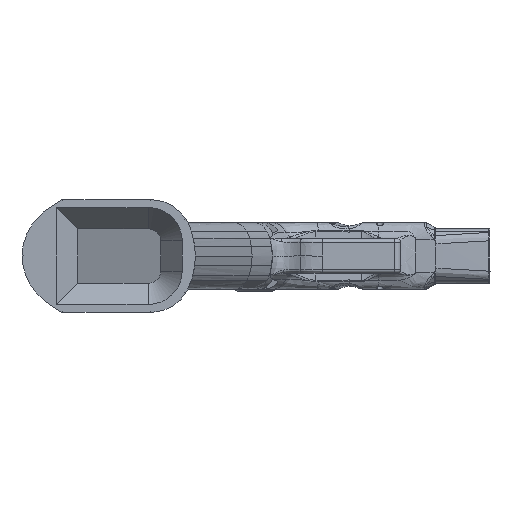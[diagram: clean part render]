
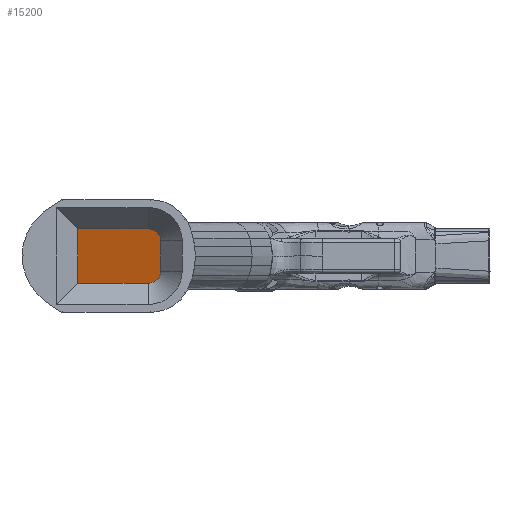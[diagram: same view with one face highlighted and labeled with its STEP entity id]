
A CAD part, front view. The second image highlights one B-rep face of the part: STEP entity #15200.
In plain terms, the highlighted planar face has unit normal (0.951, -0.309, 0).
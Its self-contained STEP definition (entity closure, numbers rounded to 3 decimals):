
#685 = CARTESIAN_POINT ( 'NONE',  ( 32.169, -5.875, -11.75 ) ) ;
#763 = EDGE_CURVE ( 'NONE', #20074, #12937, #11193, .T. ) ;
#1155 = VECTOR ( 'NONE', #11924, 1000. ) ;
#1711 = VECTOR ( 'NONE', #37430, 1000. ) ;
#1753 = LINE ( 'NONE', #5412, #18386 ) ;
#2363 = ORIENTED_EDGE ( 'NONE', *, *, #28812, .F. ) ;
#2663 = CARTESIAN_POINT ( 'NONE',  ( 32.169, -5.875, -11.75 ) ) ;
#3566 = VERTEX_POINT ( 'NONE', #685 ) ;
#4334 = VERTEX_POINT ( 'NONE', #40882 ) ;
#5311 = CARTESIAN_POINT ( 'NONE',  ( -22.8, -175.052, 11.75 ) ) ;
#5412 = CARTESIAN_POINT ( 'NONE',  ( -22.8, -175.052, -11.75 ) ) ;
#7795 = CARTESIAN_POINT ( 'NONE',  ( 32.169, -5.875, -11.75 ) ) ;
#8063 = VECTOR ( 'NONE', #37398, 1000. ) ;
#8209 = DIRECTION ( 'NONE',  ( 0.309, 0.951, 0. ) ) ;
#8543 = ORIENTED_EDGE ( 'NONE', *, *, #13688, .T. ) ;
#8795 = VERTEX_POINT ( 'NONE', #20114 ) ;
#8968 = ORIENTED_EDGE ( 'NONE', *, *, #29911, .F. ) ;
#9107 = DIRECTION ( 'NONE',  ( 0., 0., 1. ) ) ;
#10800 = VECTOR ( 'NONE', #22434, 1000. ) ;
#11193 = LINE ( 'NONE', #24298, #8063 ) ;
#11903 = LINE ( 'NONE', #41331, #29871 ) ;
#11924 = DIRECTION ( 'NONE',  ( -0.309, -0.951, 0. ) ) ;
#12059 = LINE ( 'NONE', #34624, #29429 ) ;
#12372 = VERTEX_POINT ( 'NONE', #12800 ) ;
#12542 = ORIENTED_EDGE ( 'NONE', *, *, #29637, .T. ) ;
#12647 = DIRECTION ( 'NONE',  ( -0.951, 0.309, 0. ) ) ;
#12800 = CARTESIAN_POINT ( 'NONE',  ( 33.591, -1.5, -10.375 ) ) ;
#12937 = VERTEX_POINT ( 'NONE', #38001 ) ;
#13088 = CARTESIAN_POINT ( 'NONE',  ( 2.312, -97.765, -11.75 ) ) ;
#13688 = EDGE_CURVE ( 'NONE', #12372, #33228, #11903, .T. ) ;
#13911 = EDGE_CURVE ( 'NONE', #3566, #4334, #30365, .T. ) ;
#15200 = ADVANCED_FACE ( 'NONE', ( #42074 ), #42513, .F. ) ;
#16532 = ORIENTED_EDGE ( 'NONE', *, *, #13911, .F. ) ;
#16908 = VECTOR ( 'NONE', #19029, 1000. ) ;
#18386 = VECTOR ( 'NONE', #38485, 1000. ) ;
#18721 = ORIENTED_EDGE ( 'NONE', *, *, #35594, .F. ) ;
#19029 = DIRECTION ( 'NONE',  ( 0.309, 0.951, 0. ) ) ;
#20074 = VERTEX_POINT ( 'NONE', #28000 ) ;
#20114 = CARTESIAN_POINT ( 'NONE',  ( 32.169, -5.875, -10.375 ) ) ;
#21379 = LINE ( 'NONE', #38751, #1155 ) ;
#21643 = VERTEX_POINT ( 'NONE', #5311 ) ;
#22434 = DIRECTION ( 'NONE',  ( 0., 0., -1. ) ) ;
#23694 = EDGE_LOOP ( 'NONE', ( #18721, #12542, #16532, #38215, #8968, #8543, #2363, #31585 ) ) ;
#24298 = CARTESIAN_POINT ( 'NONE',  ( 30.049, -12.4, -11.75 ) ) ;
#28000 = CARTESIAN_POINT ( 'NONE',  ( 30.049, -12.4, 11.75 ) ) ;
#28812 = EDGE_CURVE ( 'NONE', #12937, #33228, #28924, .T. ) ;
#28924 = LINE ( 'NONE', #32371, #16908 ) ;
#29429 = VECTOR ( 'NONE', #8209, 1000. ) ;
#29637 = EDGE_CURVE ( 'NONE', #21643, #4334, #1753, .T. ) ;
#29871 = VECTOR ( 'NONE', #9107, 1000. ) ;
#29911 = EDGE_CURVE ( 'NONE', #12372, #8795, #21379, .T. ) ;
#30365 = LINE ( 'NONE', #7795, #1711 ) ;
#31436 = EDGE_CURVE ( 'NONE', #8795, #3566, #38753, .T. ) ;
#31585 = ORIENTED_EDGE ( 'NONE', *, *, #763, .F. ) ;
#32371 = CARTESIAN_POINT ( 'NONE',  ( 2.312, -97.765, 4.75 ) ) ;
#33147 = CARTESIAN_POINT ( 'NONE',  ( 33.591, -1.5, 4.75 ) ) ;
#33228 = VERTEX_POINT ( 'NONE', #33147 ) ;
#34624 = CARTESIAN_POINT ( 'NONE',  ( 2.312, -97.765, 11.75 ) ) ;
#35594 = EDGE_CURVE ( 'NONE', #21643, #20074, #12059, .T. ) ;
#37398 = DIRECTION ( 'NONE',  ( 0., 0., -1. ) ) ;
#37430 = DIRECTION ( 'NONE',  ( -0.309, -0.951, 0. ) ) ;
#38001 = CARTESIAN_POINT ( 'NONE',  ( 30.049, -12.4, 4.75 ) ) ;
#38215 = ORIENTED_EDGE ( 'NONE', *, *, #31436, .F. ) ;
#38485 = DIRECTION ( 'NONE',  ( 0., 0., -1. ) ) ;
#38751 = CARTESIAN_POINT ( 'NONE',  ( 2.312, -97.765, -10.375 ) ) ;
#38753 = LINE ( 'NONE', #2663, #10800 ) ;
#38854 = DIRECTION ( 'NONE',  ( -0.309, -0.951, 0. ) ) ;
#40882 = CARTESIAN_POINT ( 'NONE',  ( -22.8, -175.052, -11.75 ) ) ;
#41331 = CARTESIAN_POINT ( 'NONE',  ( 33.591, -1.5, 0. ) ) ;
#41650 = AXIS2_PLACEMENT_3D ( 'NONE', #13088, #12647, #38854 ) ;
#42074 = FACE_OUTER_BOUND ( 'NONE', #23694, .T. ) ;
#42513 = PLANE ( 'NONE',  #41650 ) ;
